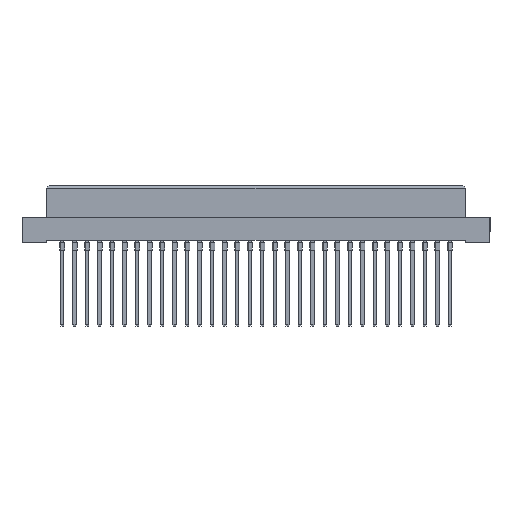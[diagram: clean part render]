
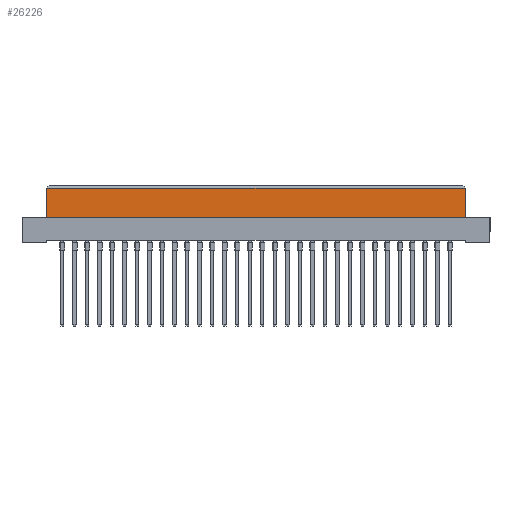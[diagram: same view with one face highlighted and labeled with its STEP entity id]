
A CAD part, top view. The second image highlights one B-rep face of the part: STEP entity #26226.
In plain terms, the highlighted planar face has unit normal (0, 0, 1).
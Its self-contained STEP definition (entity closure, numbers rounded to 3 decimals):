
#1086 = DIRECTION ( 'NONE',  ( 0., 0., 1. ) ) ;
#1636 = CARTESIAN_POINT ( 'NONE',  ( 42.5, -0.5, 4.25 ) ) ;
#3461 = VECTOR ( 'NONE', #29640, 1000. ) ;
#3556 = ORIENTED_EDGE ( 'NONE', *, *, #21195, .T. ) ;
#6015 = CARTESIAN_POINT ( 'NONE',  ( -42.5, -0.5, 4.25 ) ) ;
#7653 = CARTESIAN_POINT ( 'NONE',  ( -42.5, -6.4, 4.25 ) ) ;
#8303 = VECTOR ( 'NONE', #11317, 1000. ) ;
#9538 = CARTESIAN_POINT ( 'NONE',  ( -42.5, -6.4, 4.25 ) ) ;
#10143 = FACE_OUTER_BOUND ( 'NONE', #12822, .T. ) ;
#10856 = CARTESIAN_POINT ( 'NONE',  ( -42.5, -0.5, 4.25 ) ) ;
#11317 = DIRECTION ( 'NONE',  ( 0., 1., 0. ) ) ;
#12725 = DIRECTION ( 'NONE',  ( 1., 0., 0. ) ) ;
#12822 = EDGE_LOOP ( 'NONE', ( #3556, #37960, #25400, #24168 ) ) ;
#14265 = VECTOR ( 'NONE', #34267, 1000. ) ;
#15117 = EDGE_CURVE ( 'NONE', #18553, #32116, #22131, .T. ) ;
#17168 = CARTESIAN_POINT ( 'NONE',  ( 42.5, -6.4, 4.25 ) ) ;
#17637 = LINE ( 'NONE', #6015, #3461 ) ;
#18553 = VERTEX_POINT ( 'NONE', #7653 ) ;
#19900 = VERTEX_POINT ( 'NONE', #17168 ) ;
#20373 = CARTESIAN_POINT ( 'NONE',  ( 42.5, -6.4, 4.25 ) ) ;
#21195 = EDGE_CURVE ( 'NONE', #19900, #30392, #26474, .T. ) ;
#22131 = LINE ( 'NONE', #9538, #30100 ) ;
#24168 = ORIENTED_EDGE ( 'NONE', *, *, #36856, .T. ) ;
#25282 = DIRECTION ( 'NONE',  ( 0., 1., 0. ) ) ;
#25400 = ORIENTED_EDGE ( 'NONE', *, *, #15117, .F. ) ;
#26226 = ADVANCED_FACE ( 'NONE', ( #10143 ), #33607, .T. ) ;
#26474 = LINE ( 'NONE', #20373, #8303 ) ;
#27693 = CARTESIAN_POINT ( 'NONE',  ( 42.5, -6.4, 4.25 ) ) ;
#29640 = DIRECTION ( 'NONE',  ( -1., 0., 0. ) ) ;
#30100 = VECTOR ( 'NONE', #25282, 1000. ) ;
#30392 = VERTEX_POINT ( 'NONE', #1636 ) ;
#32116 = VERTEX_POINT ( 'NONE', #10856 ) ;
#33086 = EDGE_CURVE ( 'NONE', #30392, #32116, #17637, .T. ) ;
#33607 = PLANE ( 'NONE',  #36719 ) ;
#34267 = DIRECTION ( 'NONE',  ( 1., 0., 0. ) ) ;
#36719 = AXIS2_PLACEMENT_3D ( 'NONE', #27693, #1086, #12725 ) ;
#36856 = EDGE_CURVE ( 'NONE', #18553, #19900, #37406, .T. ) ;
#37406 = LINE ( 'NONE', #37800, #14265 ) ;
#37800 = CARTESIAN_POINT ( 'NONE',  ( 42.5, -6.4, 4.25 ) ) ;
#37960 = ORIENTED_EDGE ( 'NONE', *, *, #33086, .T. ) ;
